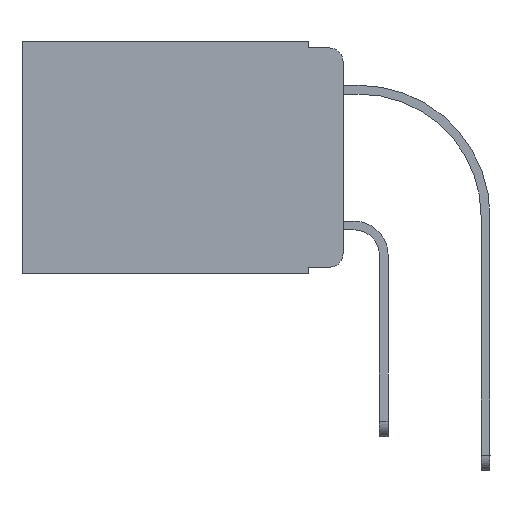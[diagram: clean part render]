
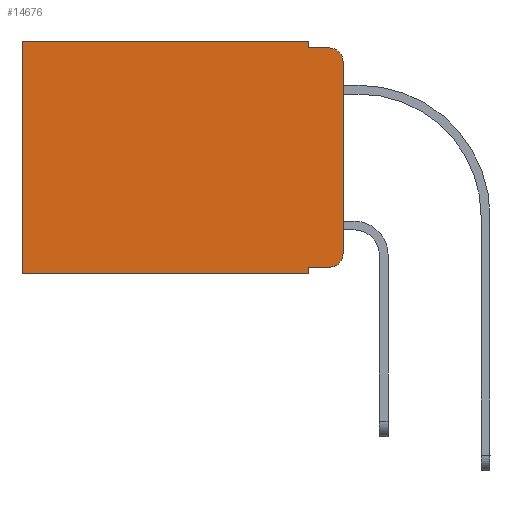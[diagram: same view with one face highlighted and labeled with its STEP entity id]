
A CAD part, left-side view. The second image highlights one B-rep face of the part: STEP entity #14676.
In plain terms, the highlighted planar face has unit normal (-1, 0, 0).
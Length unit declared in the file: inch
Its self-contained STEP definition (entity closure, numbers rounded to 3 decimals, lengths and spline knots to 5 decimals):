
#143 = PLANE ( 'NONE',  #4704 ) ;
#218 = EDGE_LOOP ( 'NONE', ( #2245, #5725, #682, #10854, #2111, #20973, #25987, #25565, #24833, #25764 ) ) ;
#682 = ORIENTED_EDGE ( 'NONE', *, *, #11324, .F. ) ;
#691 = EDGE_CURVE ( 'NONE', #17325, #20460, #19612, .T. ) ;
#960 = CARTESIAN_POINT ( 'NONE',  ( 0.298, 0., 0. ) ) ;
#1085 = CARTESIAN_POINT ( 'NONE',  ( 0.298, 0.051, 0. ) ) ;
#1198 = CIRCLE ( 'NONE', #9989, 0.02 ) ;
#1923 = DIRECTION ( 'NONE',  ( 1., 0., 0. ) ) ;
#2061 = DIRECTION ( 'NONE',  ( 0., 1., 0. ) ) ;
#2111 = ORIENTED_EDGE ( 'NONE', *, *, #15890, .T. ) ;
#2245 = ORIENTED_EDGE ( 'NONE', *, *, #4355, .F. ) ;
#2479 = EDGE_CURVE ( 'NONE', #8029, #24343, #20974, .T. ) ;
#2681 = VERTEX_POINT ( 'NONE', #12555 ) ;
#2731 = VECTOR ( 'NONE', #26888, 39.37008 ) ;
#3144 = CARTESIAN_POINT ( 'NONE',  ( 0.298, 0.051, -0.343 ) ) ;
#3696 = CARTESIAN_POINT ( 'NONE',  ( 0.298, 0.473, -0.343 ) ) ;
#3838 = CARTESIAN_POINT ( 'NONE',  ( 0.298, 0.02, -0.333 ) ) ;
#4118 = CARTESIAN_POINT ( 'NONE',  ( 0.298, 0.02, -0.01 ) ) ;
#4127 = CARTESIAN_POINT ( 'NONE',  ( 0.298, 0.02, -0.313 ) ) ;
#4355 = EDGE_CURVE ( 'NONE', #17498, #7944, #15738, .T. ) ;
#4704 = AXIS2_PLACEMENT_3D ( 'NONE', #6178, #1923, #25328 ) ;
#4878 = EDGE_CURVE ( 'NONE', #17325, #24635, #18125, .T. ) ;
#5725 = ORIENTED_EDGE ( 'NONE', *, *, #14190, .T. ) ;
#5830 = LINE ( 'NONE', #26768, #9354 ) ;
#6178 = CARTESIAN_POINT ( 'NONE',  ( 0.298, 0., 0. ) ) ;
#6376 = CARTESIAN_POINT ( 'NONE',  ( 0.298, 0.051, -0.01 ) ) ;
#6430 = LINE ( 'NONE', #10137, #16928 ) ;
#6789 = VERTEX_POINT ( 'NONE', #4118 ) ;
#6873 = DIRECTION ( 'NONE',  ( 0., 0., -1. ) ) ;
#7944 = VERTEX_POINT ( 'NONE', #11556 ) ;
#8029 = VERTEX_POINT ( 'NONE', #15783 ) ;
#8705 = DIRECTION ( 'NONE',  ( 0., -1., 0. ) ) ;
#9354 = VECTOR ( 'NONE', #24186, 39.37008 ) ;
#9989 = AXIS2_PLACEMENT_3D ( 'NONE', #12931, #12662, #25392 ) ;
#10137 = CARTESIAN_POINT ( 'NONE',  ( 0.298, 0.051, 0. ) ) ;
#10405 = FACE_OUTER_BOUND ( 'NONE', #218, .T. ) ;
#10536 = DIRECTION ( 'NONE',  ( 0., 0., -1. ) ) ;
#10854 = ORIENTED_EDGE ( 'NONE', *, *, #19290, .F. ) ;
#10942 = CARTESIAN_POINT ( 'NONE',  ( 0.298, 0., -0.03 ) ) ;
#11324 = EDGE_CURVE ( 'NONE', #2681, #6789, #15119, .T. ) ;
#11556 = CARTESIAN_POINT ( 'NONE',  ( 0.298, 0., -0.313 ) ) ;
#12555 = CARTESIAN_POINT ( 'NONE',  ( 0.298, 0.051, -0.01 ) ) ;
#12662 = DIRECTION ( 'NONE',  ( -1., 0., 0. ) ) ;
#12931 = CARTESIAN_POINT ( 'NONE',  ( 0.298, 0.02, -0.03 ) ) ;
#13562 = DIRECTION ( 'NONE',  ( 0., 0., -1. ) ) ;
#13985 = VECTOR ( 'NONE', #8705, 39.37008 ) ;
#14166 = CARTESIAN_POINT ( 'NONE',  ( 0.298, 0.051, 0. ) ) ;
#14190 = EDGE_CURVE ( 'NONE', #17498, #6789, #1198, .T. ) ;
#14525 = LINE ( 'NONE', #20800, #24009 ) ;
#14676 = ADVANCED_FACE ( 'NONE', ( #10405 ), #143, .F. ) ;
#15119 = LINE ( 'NONE', #6376, #13985 ) ;
#15738 = LINE ( 'NONE', #960, #22803 ) ;
#15783 = CARTESIAN_POINT ( 'NONE',  ( 0.298, 0.473, 0. ) ) ;
#15814 = DIRECTION ( 'NONE',  ( -1., 0., 0. ) ) ;
#15890 = EDGE_CURVE ( 'NONE', #19644, #8029, #14525, .T. ) ;
#16443 = DIRECTION ( 'NONE',  ( 0., 0., -1. ) ) ;
#16928 = VECTOR ( 'NONE', #10536, 39.37008 ) ;
#16961 = EDGE_CURVE ( 'NONE', #20460, #7944, #17034, .T. ) ;
#17034 = CIRCLE ( 'NONE', #20961, 0.02 ) ;
#17325 = VERTEX_POINT ( 'NONE', #18466 ) ;
#17498 = VERTEX_POINT ( 'NONE', #10942 ) ;
#17976 = CARTESIAN_POINT ( 'NONE',  ( 0.298, 0.051, -0.333 ) ) ;
#18125 = LINE ( 'NONE', #14166, #2731 ) ;
#18466 = CARTESIAN_POINT ( 'NONE',  ( 0.298, 0.051, -0.333 ) ) ;
#19290 = EDGE_CURVE ( 'NONE', #19644, #2681, #6430, .T. ) ;
#19612 = LINE ( 'NONE', #17976, #24408 ) ;
#19644 = VERTEX_POINT ( 'NONE', #1085 ) ;
#20460 = VERTEX_POINT ( 'NONE', #3838 ) ;
#20800 = CARTESIAN_POINT ( 'NONE',  ( 0.298, 0., 0. ) ) ;
#20961 = AXIS2_PLACEMENT_3D ( 'NONE', #4127, #15814, #16443 ) ;
#20973 = ORIENTED_EDGE ( 'NONE', *, *, #2479, .T. ) ;
#20974 = LINE ( 'NONE', #23989, #25249 ) ;
#22803 = VECTOR ( 'NONE', #13562, 39.37008 ) ;
#23989 = CARTESIAN_POINT ( 'NONE',  ( 0.298, 0.473, 0. ) ) ;
#24009 = VECTOR ( 'NONE', #2061, 39.37008 ) ;
#24186 = DIRECTION ( 'NONE',  ( 0., 1., 0. ) ) ;
#24269 = DIRECTION ( 'NONE',  ( 0., -1., 0. ) ) ;
#24343 = VERTEX_POINT ( 'NONE', #3696 ) ;
#24408 = VECTOR ( 'NONE', #24269, 39.37008 ) ;
#24635 = VERTEX_POINT ( 'NONE', #3144 ) ;
#24833 = ORIENTED_EDGE ( 'NONE', *, *, #691, .T. ) ;
#25249 = VECTOR ( 'NONE', #6873, 39.37008 ) ;
#25328 = DIRECTION ( 'NONE',  ( 0., 0., -1. ) ) ;
#25392 = DIRECTION ( 'NONE',  ( 0., 0., -1. ) ) ;
#25565 = ORIENTED_EDGE ( 'NONE', *, *, #4878, .F. ) ;
#25764 = ORIENTED_EDGE ( 'NONE', *, *, #16961, .T. ) ;
#25987 = ORIENTED_EDGE ( 'NONE', *, *, #26593, .F. ) ;
#26593 = EDGE_CURVE ( 'NONE', #24635, #24343, #5830, .T. ) ;
#26768 = CARTESIAN_POINT ( 'NONE',  ( 0.298, 0., -0.343 ) ) ;
#26888 = DIRECTION ( 'NONE',  ( 0., 0., -1. ) ) ;
